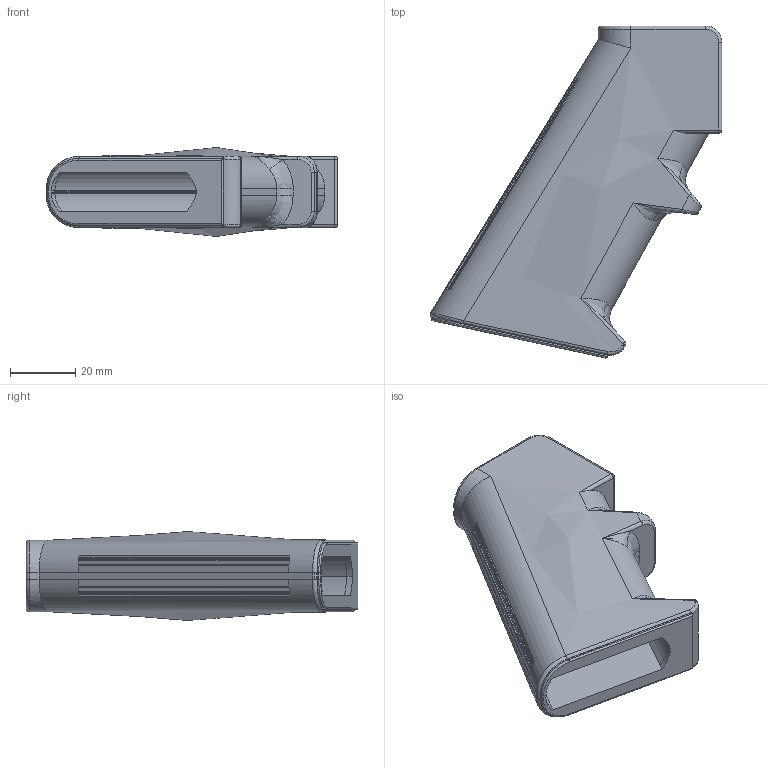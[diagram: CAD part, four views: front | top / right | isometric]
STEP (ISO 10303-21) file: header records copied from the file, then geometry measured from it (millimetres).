
FILE_DESCRIPTION (( 'STEP AP214' ), '1' );
FILE_NAME ('AR-15_Grip.STEP', '2013-09-21T05:25:13', ( 'elpi' ), ( '' ), 'SwSTEP 2.0', 'SolidWorks 2013', '' );
FILE_SCHEMA (( 'AUTOMOTIVE_DESIGN' ));
Length unit declared in the file: millimetre
Products named in the file (1): AR-15_Grip
Bounding box: 89.68 x 102.1 x 27.36 mm (x, y, z)
Volume: 58984 mm3; surface area: 25509.9 mm2
Topology: 1 solids, 1 shells, 171 faces, 409 edges, 240 vertices
Faces by surface type: plane 60, cylinder 53, bspline 50, torus 4, sphere 4
Entity records: 8638 total; most frequent: CARTESIAN_POINT 5160, ORIENTED_EDGE 794, DIRECTION 603, EDGE_CURVE 397, VERTEX_POINT 238, AXIS2_PLACEMENT_3D 216, EDGE_LOOP 183, FACE_OUTER_BOUND 171
